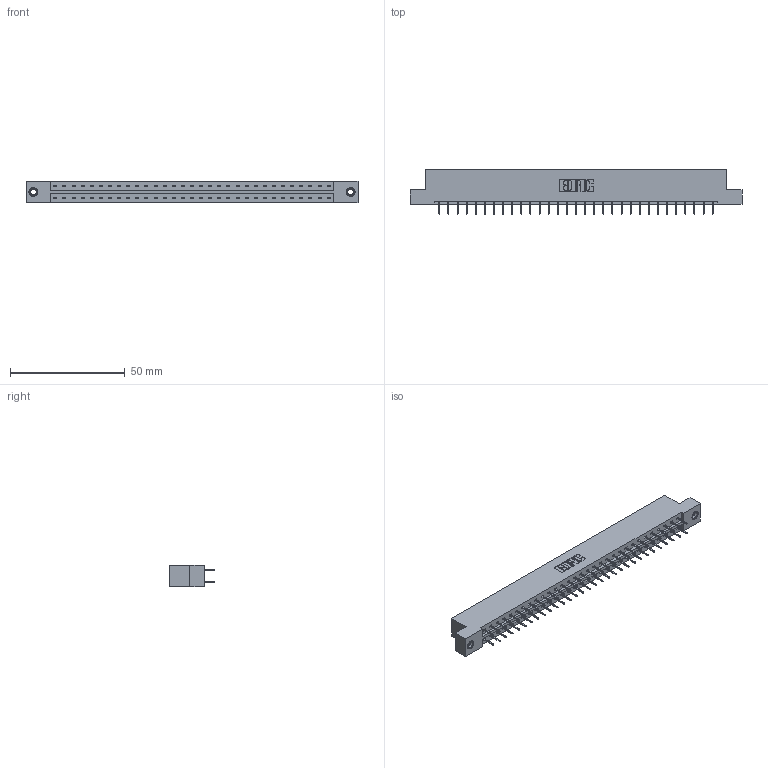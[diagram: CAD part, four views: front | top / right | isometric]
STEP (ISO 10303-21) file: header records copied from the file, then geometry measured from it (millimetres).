
FILE_DESCRIPTION (( 'STEP AP203' ), '1' );
FILE_NAME ('833-062-524-207.STEP', '2020-06-05T05:26:58', ( '' ), ( '' ), 'SwSTEP 2.0', 'SolidWorks 2020', '' );
FILE_SCHEMA (( 'CONFIG_CONTROL_DESIGN' ));
Length unit declared in the file: inch
Products named in the file (4): 345-292-001_345-293-124; 833-062-524-207; 345-250-001_345-250-005-103; 833 Part_Flush - .156 Dia - TI
Assembly tree (65 placements, depth 2):
  833-062-524-207
    833 Part_Flush - .156 Dia - TI
    345-292-001_345-293-124  x62
    345-250-001_345-250-005-103  x2
Bounding box: 144.37 x 19.69 x 9.4 mm (x, y, z)
Volume: 14529.5 mm3; surface area: 16811.8 mm2
Topology: 65 solids, 65 shells, 3646 faces, 10305 edges, 6614 vertices
Faces by surface type: plane 2706, cylinder 924, cone 12, torus 4
Entity records: 22626 total; most frequent: CARTESIAN_POINT 3745, ORIENTED_EDGE 3674, DIRECTION 3251, EDGE_CURVE 1837, VECTOR 1693, LINE 1693, VERTEX_POINT 1216, AXIS2_PLACEMENT_3D 779
